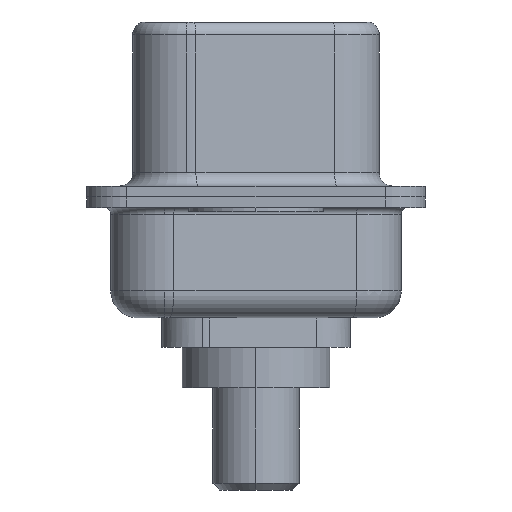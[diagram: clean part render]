
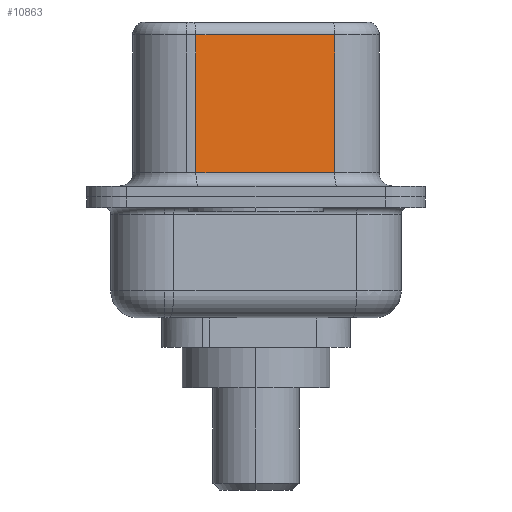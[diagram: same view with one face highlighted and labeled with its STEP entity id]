
A CAD part, left-side view. The second image highlights one B-rep face of the part: STEP entity #10863.
In plain terms, the highlighted planar face has unit normal (-0.985, -0.174, 0).
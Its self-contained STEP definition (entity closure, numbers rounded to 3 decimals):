
#97 = PLANE ( 'NONE',  #2659 ) ;
#272 = VERTEX_POINT ( 'NONE', #1510 ) ;
#278 = DIRECTION ( 'NONE',  ( 0., 0., -1. ) ) ;
#466 = DIRECTION ( 'NONE',  ( -0.174, 0.985, 0. ) ) ;
#486 = CARTESIAN_POINT ( 'NONE',  ( 4.565, -2.927, 0.9 ) ) ;
#758 = ORIENTED_EDGE ( 'NONE', *, *, #9951, .T. ) ;
#802 = DIRECTION ( 'NONE',  ( 0., 0., -1. ) ) ;
#884 = FACE_OUTER_BOUND ( 'NONE', #6769, .T. ) ;
#948 = CARTESIAN_POINT ( 'NONE',  ( 3.655, 2.233, 0.9 ) ) ;
#1206 = EDGE_CURVE ( 'NONE', #5296, #4491, #3663, .T. ) ;
#1510 = CARTESIAN_POINT ( 'NONE',  ( 4.565, -2.927, 0.9 ) ) ;
#1720 = CARTESIAN_POINT ( 'NONE',  ( 4.565, -2.927, 6.52 ) ) ;
#1802 = DIRECTION ( 'NONE',  ( 0.985, 0.174, 0. ) ) ;
#2046 = DIRECTION ( 'NONE',  ( 0.174, -0.985, 0. ) ) ;
#2210 = ORIENTED_EDGE ( 'NONE', *, *, #8404, .T. ) ;
#2240 = VECTOR ( 'NONE', #802, 1000. ) ;
#2659 = AXIS2_PLACEMENT_3D ( 'NONE', #1720, #1802, #9498 ) ;
#3008 = VECTOR ( 'NONE', #466, 1000. ) ;
#3349 = CARTESIAN_POINT ( 'NONE',  ( 4.565, -2.927, 6.52 ) ) ;
#3663 = LINE ( 'NONE', #6327, #3008 ) ;
#4120 = VECTOR ( 'NONE', #278, 1000. ) ;
#4491 = VERTEX_POINT ( 'NONE', #6823 ) ;
#5069 = LINE ( 'NONE', #10355, #4120 ) ;
#5296 = VERTEX_POINT ( 'NONE', #7871 ) ;
#6191 = ORIENTED_EDGE ( 'NONE', *, *, #10224, .F. ) ;
#6327 = CARTESIAN_POINT ( 'NONE',  ( 4.565, -2.927, 6.02 ) ) ;
#6769 = EDGE_LOOP ( 'NONE', ( #6191, #8747, #2210, #758 ) ) ;
#6823 = CARTESIAN_POINT ( 'NONE',  ( 3.655, 2.233, 6.02 ) ) ;
#7641 = VECTOR ( 'NONE', #2046, 1000. ) ;
#7871 = CARTESIAN_POINT ( 'NONE',  ( 4.565, -2.927, 6.02 ) ) ;
#8404 = EDGE_CURVE ( 'NONE', #4491, #10294, #5069, .T. ) ;
#8560 = LINE ( 'NONE', #486, #7641 ) ;
#8697 = LINE ( 'NONE', #3349, #2240 ) ;
#8747 = ORIENTED_EDGE ( 'NONE', *, *, #1206, .T. ) ;
#9498 = DIRECTION ( 'NONE',  ( -0.174, 0.985, 0. ) ) ;
#9951 = EDGE_CURVE ( 'NONE', #10294, #272, #8560, .T. ) ;
#10224 = EDGE_CURVE ( 'NONE', #5296, #272, #8697, .T. ) ;
#10294 = VERTEX_POINT ( 'NONE', #948 ) ;
#10355 = CARTESIAN_POINT ( 'NONE',  ( 3.655, 2.233, 6.52 ) ) ;
#10863 = ADVANCED_FACE ( 'NONE', ( #884 ), #97, .F. ) ;
